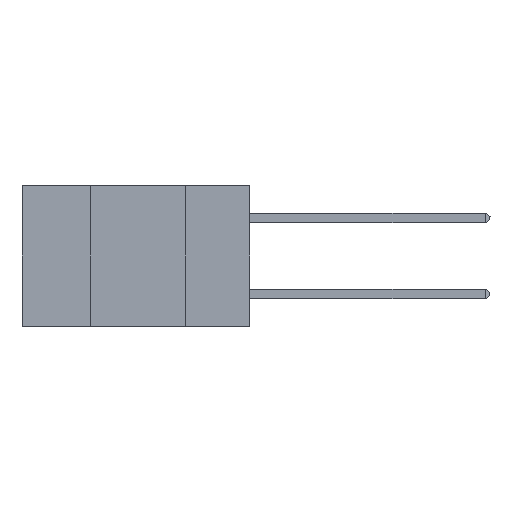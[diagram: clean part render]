
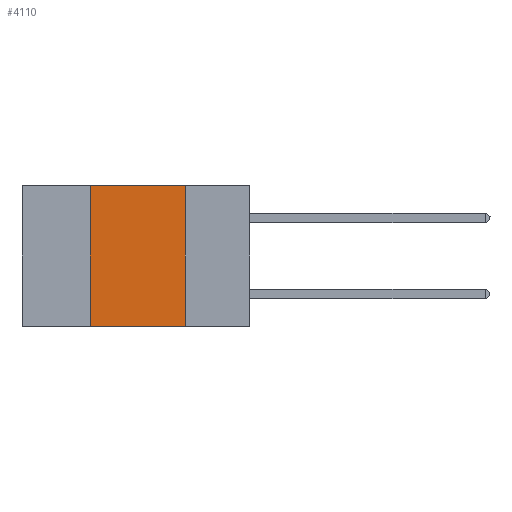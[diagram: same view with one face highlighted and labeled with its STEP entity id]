
A CAD part, left-side view. The second image highlights one B-rep face of the part: STEP entity #4110.
In plain terms, the highlighted planar face has unit normal (-1, 0, 0).
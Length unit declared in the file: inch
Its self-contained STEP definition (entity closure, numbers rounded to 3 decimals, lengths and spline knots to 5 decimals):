
#454 = VERTEX_POINT ( 'NONE', #16954 ) ;
#680 = DIRECTION ( 'NONE',  ( 1., 0., 0. ) ) ;
#2018 = FACE_OUTER_BOUND ( 'NONE', #12375, .T. ) ;
#2283 = LINE ( 'NONE', #2967, #21481 ) ;
#2315 = VECTOR ( 'NONE', #5895, 39.37008 ) ;
#2967 = CARTESIAN_POINT ( 'NONE',  ( 0., 0.6, 0. ) ) ;
#3517 = ORIENTED_EDGE ( 'NONE', *, *, #11239, .T. ) ;
#4110 = ADVANCED_FACE ( 'NONE', ( #2018 ), #18158, .F. ) ;
#4314 = EDGE_CURVE ( 'NONE', #18689, #454, #2283, .T. ) ;
#5367 = LINE ( 'NONE', #9209, #14206 ) ;
#5895 = DIRECTION ( 'NONE',  ( 0., 0., -1. ) ) ;
#6413 = EDGE_CURVE ( 'NONE', #22628, #18689, #20601, .T. ) ;
#6832 = DIRECTION ( 'NONE',  ( 0., 0., 1. ) ) ;
#7837 = ORIENTED_EDGE ( 'NONE', *, *, #4314, .F. ) ;
#9052 = CARTESIAN_POINT ( 'NONE',  ( 0., 0.42, 0. ) ) ;
#9209 = CARTESIAN_POINT ( 'NONE',  ( 0., 0.6, -0.37 ) ) ;
#10980 = DIRECTION ( 'NONE',  ( 0., -1., 0. ) ) ;
#11239 = EDGE_CURVE ( 'NONE', #22628, #20883, #5367, .T. ) ;
#12375 = EDGE_LOOP ( 'NONE', ( #21014, #7837, #21532, #3517 ) ) ;
#13439 = CARTESIAN_POINT ( 'NONE',  ( 0., 0.17, -0.37 ) ) ;
#14206 = VECTOR ( 'NONE', #10980, 39.37008 ) ;
#15191 = CARTESIAN_POINT ( 'NONE',  ( 0., 0.42, -0.37 ) ) ;
#16373 = CARTESIAN_POINT ( 'NONE',  ( 0., 0.17, 0. ) ) ;
#16709 = DIRECTION ( 'NONE',  ( 0., -1., 0. ) ) ;
#16954 = CARTESIAN_POINT ( 'NONE',  ( 0., 0.17, 0. ) ) ;
#17239 = CARTESIAN_POINT ( 'NONE',  ( 0., 0.42, 0. ) ) ;
#18158 = PLANE ( 'NONE',  #18745 ) ;
#18689 = VERTEX_POINT ( 'NONE', #9052 ) ;
#18745 = AXIS2_PLACEMENT_3D ( 'NONE', #22050, #680, #22370 ) ;
#20054 = EDGE_CURVE ( 'NONE', #454, #20883, #20989, .T. ) ;
#20601 = LINE ( 'NONE', #17239, #21121 ) ;
#20883 = VERTEX_POINT ( 'NONE', #13439 ) ;
#20989 = LINE ( 'NONE', #16373, #2315 ) ;
#21014 = ORIENTED_EDGE ( 'NONE', *, *, #20054, .F. ) ;
#21121 = VECTOR ( 'NONE', #6832, 39.37008 ) ;
#21481 = VECTOR ( 'NONE', #16709, 39.37008 ) ;
#21532 = ORIENTED_EDGE ( 'NONE', *, *, #6413, .F. ) ;
#22050 = CARTESIAN_POINT ( 'NONE',  ( 0., 0.6, 0. ) ) ;
#22370 = DIRECTION ( 'NONE',  ( 0., 0., -1. ) ) ;
#22628 = VERTEX_POINT ( 'NONE', #15191 ) ;
